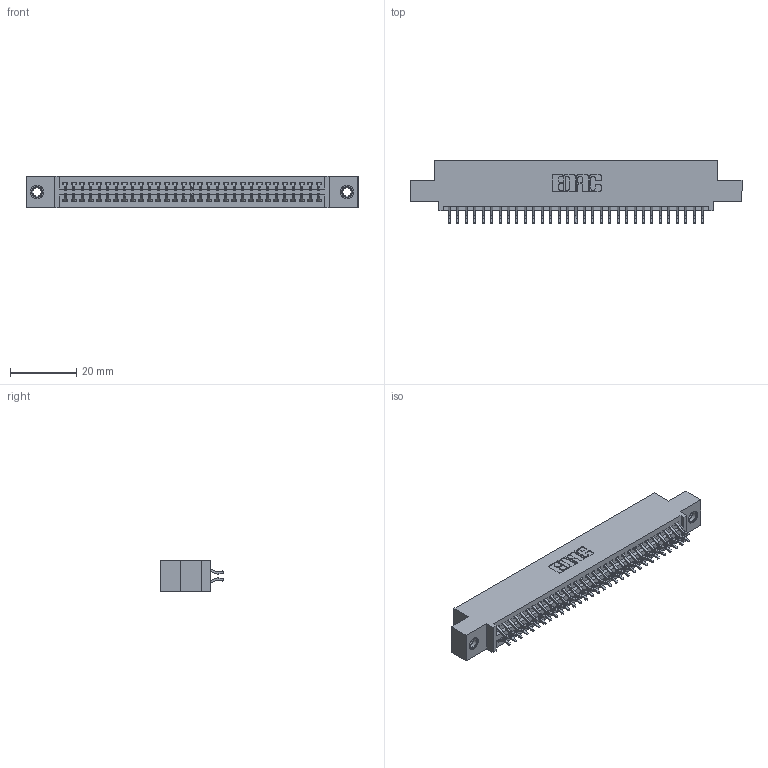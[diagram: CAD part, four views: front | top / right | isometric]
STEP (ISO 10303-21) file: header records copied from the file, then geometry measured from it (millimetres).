
FILE_DESCRIPTION (( 'STEP AP203' ), '1' );
FILE_NAME ('345-062-556-507.STEP', '2019-10-30T12:13:44', ( '' ), ( '' ), 'SwSTEP 2.0', 'SolidWorks 2016', '' );
FILE_SCHEMA (( 'CONFIG_CONTROL_DESIGN' ));
Length unit declared in the file: inch
Products named in the file (4): 345-062-556-507; 345 Part_0.110 Offset - 0.156 Dia-TI; 345-292-001_556 Tail; 345-250-001_345-250-005-103
Assembly tree (65 placements, depth 2):
  345-062-556-507
    345 Part_0.110 Offset - 0.156 Dia-TI
    345-292-001_556 Tail  x62
    345-250-001_345-250-005-103  x2
Bounding box: 99.95 x 19.24 x 9.4 mm (x, y, z)
Volume: 9517.7 mm3; surface area: 13922.2 mm2
Topology: 65 solids, 65 shells, 3662 faces, 10843 edges, 7138 vertices
Faces by surface type: plane 2410, cylinder 1236, cone 12, torus 4
Entity records: 27342 total; most frequent: CARTESIAN_POINT 4591, ORIENTED_EDGE 4506, DIRECTION 4075, EDGE_CURVE 2253, VECTOR 1969, LINE 1969, VERTEX_POINT 1496, AXIS2_PLACEMENT_3D 1053
